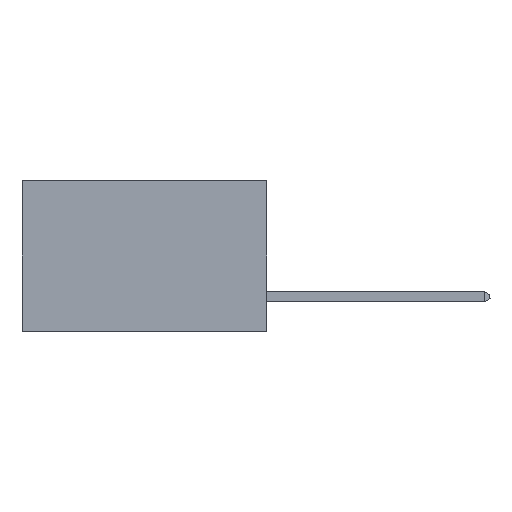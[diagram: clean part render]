
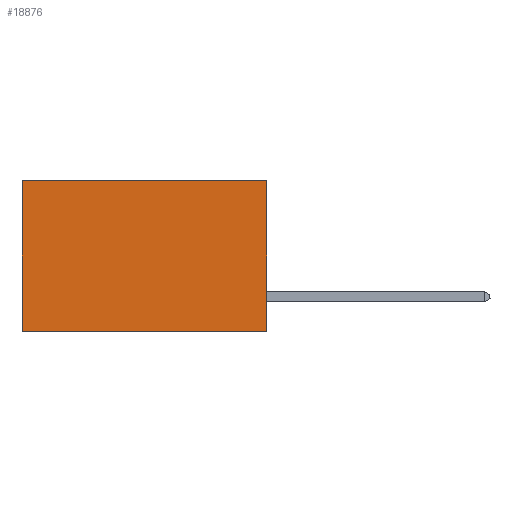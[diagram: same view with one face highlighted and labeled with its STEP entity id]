
A CAD part, left-side view. The second image highlights one B-rep face of the part: STEP entity #18876.
In plain terms, the highlighted planar face has unit normal (-1, 0, 0).
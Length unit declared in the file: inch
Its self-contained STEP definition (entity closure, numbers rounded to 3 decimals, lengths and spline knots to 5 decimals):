
#599 = DIRECTION ( 'NONE',  ( 0., 0., -1. ) ) ;
#1258 = CARTESIAN_POINT ( 'NONE',  ( 0.2875, 0., 0. ) ) ;
#2088 = CARTESIAN_POINT ( 'NONE',  ( 0.2875, 0.6, 0. ) ) ;
#2672 = DIRECTION ( 'NONE',  ( 0., 1., 0. ) ) ;
#3980 = LINE ( 'NONE', #15694, #15484 ) ;
#4160 = LINE ( 'NONE', #1258, #15023 ) ;
#4697 = CARTESIAN_POINT ( 'NONE',  ( 0.2875, 0.6, 0. ) ) ;
#5005 = ORIENTED_EDGE ( 'NONE', *, *, #19459, .T. ) ;
#5147 = LINE ( 'NONE', #4697, #21462 ) ;
#5170 = VERTEX_POINT ( 'NONE', #20206 ) ;
#6984 = DIRECTION ( 'NONE',  ( 0., 1., 0. ) ) ;
#7312 = ORIENTED_EDGE ( 'NONE', *, *, #7673, .F. ) ;
#7673 = EDGE_CURVE ( 'NONE', #25869, #21337, #23834, .T. ) ;
#7858 = VECTOR ( 'NONE', #6984, 39.37008 ) ;
#10478 = EDGE_CURVE ( 'NONE', #16011, #21337, #5147, .T. ) ;
#11418 = DIRECTION ( 'NONE',  ( 0., 0., -1. ) ) ;
#11489 = CARTESIAN_POINT ( 'NONE',  ( 0.2875, 0., -0.37 ) ) ;
#13831 = DIRECTION ( 'NONE',  ( 1., 0., 0. ) ) ;
#14649 = ORIENTED_EDGE ( 'NONE', *, *, #16409, .F. ) ;
#15023 = VECTOR ( 'NONE', #22633, 39.37008 ) ;
#15484 = VECTOR ( 'NONE', #2672, 39.37008 ) ;
#15694 = CARTESIAN_POINT ( 'NONE',  ( 0.2875, 0., 0. ) ) ;
#16011 = VERTEX_POINT ( 'NONE', #2088 ) ;
#16409 = EDGE_CURVE ( 'NONE', #5170, #25869, #4160, .T. ) ;
#17485 = CARTESIAN_POINT ( 'NONE',  ( 0.2875, 0.6, -0.37 ) ) ;
#17906 = PLANE ( 'NONE',  #22865 ) ;
#18876 = ADVANCED_FACE ( 'NONE', ( #24891 ), #17906, .F. ) ;
#19244 = ORIENTED_EDGE ( 'NONE', *, *, #10478, .T. ) ;
#19459 = EDGE_CURVE ( 'NONE', #5170, #16011, #3980, .T. ) ;
#20206 = CARTESIAN_POINT ( 'NONE',  ( 0.2875, 0., 0. ) ) ;
#21337 = VERTEX_POINT ( 'NONE', #17485 ) ;
#21462 = VECTOR ( 'NONE', #11418, 39.37008 ) ;
#22633 = DIRECTION ( 'NONE',  ( 0., 0., -1. ) ) ;
#22865 = AXIS2_PLACEMENT_3D ( 'NONE', #26190, #13831, #599 ) ;
#23834 = LINE ( 'NONE', #11489, #7858 ) ;
#24891 = FACE_OUTER_BOUND ( 'NONE', #24963, .T. ) ;
#24963 = EDGE_LOOP ( 'NONE', ( #19244, #7312, #14649, #5005 ) ) ;
#25252 = CARTESIAN_POINT ( 'NONE',  ( 0.2875, 0., -0.37 ) ) ;
#25869 = VERTEX_POINT ( 'NONE', #25252 ) ;
#26190 = CARTESIAN_POINT ( 'NONE',  ( 0.2875, 0., 0. ) ) ;
